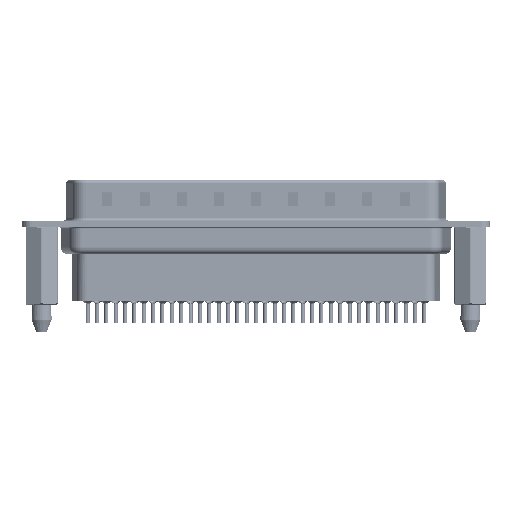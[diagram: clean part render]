
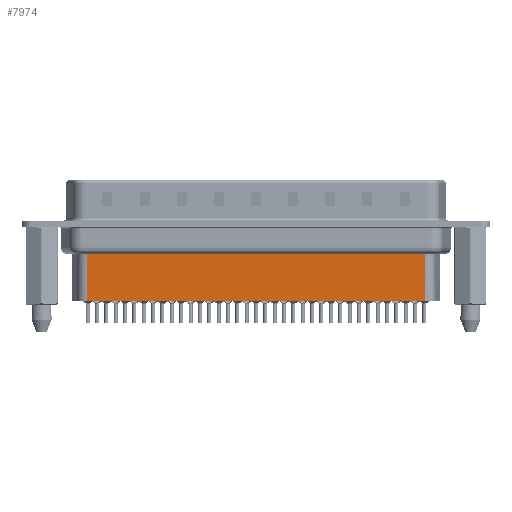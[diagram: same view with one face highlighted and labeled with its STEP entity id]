
A CAD part, front view. The second image highlights one B-rep face of the part: STEP entity #7974.
In plain terms, the highlighted planar face has unit normal (0, -1, 0).
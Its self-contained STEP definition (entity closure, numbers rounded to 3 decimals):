
#2078 = LINE ( 'NONE', #15020, #27709 ) ;
#2589 = CARTESIAN_POINT ( 'NONE',  ( 6.706, -3.5, -3.1 ) ) ;
#3131 = LINE ( 'NONE', #9171, #16303 ) ;
#4691 = VECTOR ( 'NONE', #21230, 1000. ) ;
#5080 = DIRECTION ( 'NONE',  ( 1., 0., 0. ) ) ;
#5158 = DIRECTION ( 'NONE',  ( 0., 0., -1. ) ) ;
#5677 = DIRECTION ( 'NONE',  ( -1., 0., 0. ) ) ;
#7974 = ADVANCED_FACE ( 'NONE', ( #24283 ), #12478, .T. ) ;
#8564 = EDGE_CURVE ( 'NONE', #30633, #15017, #2078, .T. ) ;
#9017 = VECTOR ( 'NONE', #5677, 1000. ) ;
#9171 = CARTESIAN_POINT ( 'NONE',  ( 6.706, -3.5, -11.45 ) ) ;
#9320 = ORIENTED_EDGE ( 'NONE', *, *, #11514, .F. ) ;
#11458 = EDGE_CURVE ( 'NONE', #14856, #11461, #24513, .T. ) ;
#11461 = VERTEX_POINT ( 'NONE', #23830 ) ;
#11514 = EDGE_CURVE ( 'NONE', #15017, #11461, #3131, .T. ) ;
#12155 = EDGE_LOOP ( 'NONE', ( #24735, #22360, #23729, #9320 ) ) ;
#12478 = PLANE ( 'NONE',  #25606 ) ;
#14856 = VERTEX_POINT ( 'NONE', #28671 ) ;
#15017 = VERTEX_POINT ( 'NONE', #21298 ) ;
#15020 = CARTESIAN_POINT ( 'NONE',  ( 56.794, -3.5, -3.1 ) ) ;
#16303 = VECTOR ( 'NONE', #26518, 1000. ) ;
#18719 = CARTESIAN_POINT ( 'NONE',  ( 6.706, -3.5, -3.1 ) ) ;
#19976 = DIRECTION ( 'NONE',  ( 0., -1., 0. ) ) ;
#21230 = DIRECTION ( 'NONE',  ( 0., 0., -1. ) ) ;
#21298 = CARTESIAN_POINT ( 'NONE',  ( 56.794, -3.5, -11.45 ) ) ;
#21343 = EDGE_CURVE ( 'NONE', #30633, #14856, #22257, .T. ) ;
#22257 = LINE ( 'NONE', #30408, #9017 ) ;
#22360 = ORIENTED_EDGE ( 'NONE', *, *, #21343, .T. ) ;
#23729 = ORIENTED_EDGE ( 'NONE', *, *, #11458, .T. ) ;
#23830 = CARTESIAN_POINT ( 'NONE',  ( 6.706, -3.5, -11.45 ) ) ;
#24283 = FACE_OUTER_BOUND ( 'NONE', #12155, .T. ) ;
#24513 = LINE ( 'NONE', #18719, #4691 ) ;
#24735 = ORIENTED_EDGE ( 'NONE', *, *, #8564, .F. ) ;
#25606 = AXIS2_PLACEMENT_3D ( 'NONE', #2589, #19976, #5080 ) ;
#26084 = CARTESIAN_POINT ( 'NONE',  ( 56.794, -3.5, -4.097 ) ) ;
#26518 = DIRECTION ( 'NONE',  ( -1., 0., 0. ) ) ;
#27709 = VECTOR ( 'NONE', #5158, 1000. ) ;
#28671 = CARTESIAN_POINT ( 'NONE',  ( 6.706, -3.5, -4.097 ) ) ;
#30408 = CARTESIAN_POINT ( 'NONE',  ( 6.459, -3.5, -4.097 ) ) ;
#30633 = VERTEX_POINT ( 'NONE', #26084 ) ;
